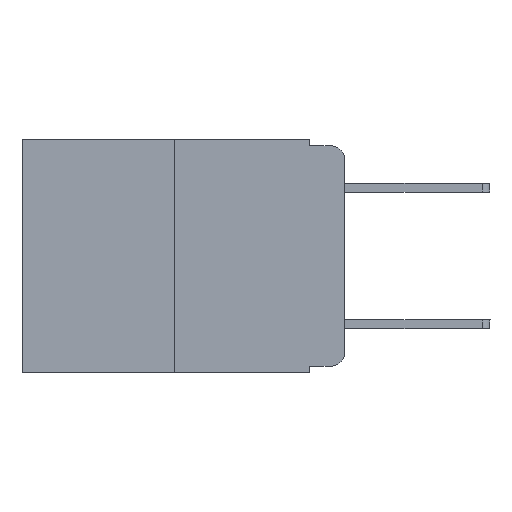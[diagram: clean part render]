
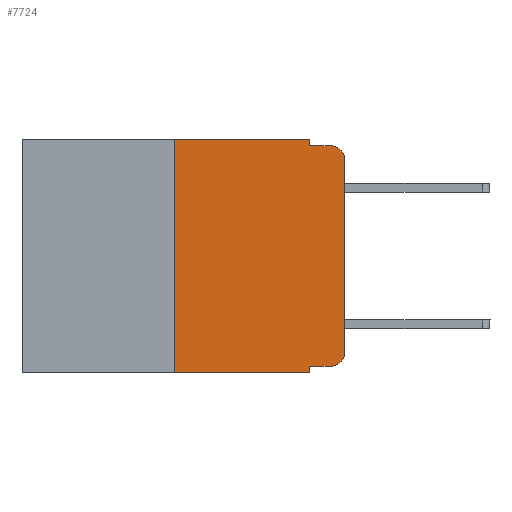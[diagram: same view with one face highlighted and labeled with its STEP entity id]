
A CAD part, left-side view. The second image highlights one B-rep face of the part: STEP entity #7724.
In plain terms, the highlighted planar face has unit normal (-1, 0, 0).
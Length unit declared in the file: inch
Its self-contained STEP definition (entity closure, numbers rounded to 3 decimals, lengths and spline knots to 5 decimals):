
#228 = CARTESIAN_POINT ( 'NONE',  ( 0., 0.02, -0.313 ) ) ;
#391 = LINE ( 'NONE', #3208, #10786 ) ;
#395 = LINE ( 'NONE', #9483, #9453 ) ;
#474 = EDGE_CURVE ( 'NONE', #6445, #5872, #391, .T. ) ;
#536 = VERTEX_POINT ( 'NONE', #8175 ) ;
#725 = DIRECTION ( 'NONE',  ( -1., 0., 0. ) ) ;
#826 = VERTEX_POINT ( 'NONE', #10182 ) ;
#1016 = ORIENTED_EDGE ( 'NONE', *, *, #15854, .T. ) ;
#1035 = VERTEX_POINT ( 'NONE', #9057 ) ;
#1087 = CARTESIAN_POINT ( 'NONE',  ( 0., 0.02, -0.01 ) ) ;
#1157 = CARTESIAN_POINT ( 'NONE',  ( 0., 0.473, -0.343 ) ) ;
#1328 = EDGE_CURVE ( 'NONE', #5872, #15276, #11912, .T. ) ;
#1641 = VERTEX_POINT ( 'NONE', #15728 ) ;
#1846 = ORIENTED_EDGE ( 'NONE', *, *, #10361, .T. ) ;
#1876 = LINE ( 'NONE', #10554, #15688 ) ;
#2297 = CARTESIAN_POINT ( 'NONE',  ( 0., 0.051, -0.01 ) ) ;
#3073 = DIRECTION ( 'NONE',  ( 1., 0., 0. ) ) ;
#3208 = CARTESIAN_POINT ( 'NONE',  ( 0., 0.25, 0. ) ) ;
#3392 = EDGE_CURVE ( 'NONE', #15276, #13575, #14019, .T. ) ;
#3909 = VECTOR ( 'NONE', #8403, 39.37008 ) ;
#4328 = DIRECTION ( 'NONE',  ( 0., 0., -1. ) ) ;
#4457 = DIRECTION ( 'NONE',  ( 0., 0., 1. ) ) ;
#4506 = DIRECTION ( 'NONE',  ( 0., -1., 0. ) ) ;
#4897 = DIRECTION ( 'NONE',  ( 0., 0., -1. ) ) ;
#4908 = EDGE_CURVE ( 'NONE', #8426, #826, #1876, .T. ) ;
#4985 = EDGE_CURVE ( 'NONE', #6445, #826, #8049, .T. ) ;
#5052 = ORIENTED_EDGE ( 'NONE', *, *, #10238, .T. ) ;
#5402 = VECTOR ( 'NONE', #4506, 39.37008 ) ;
#5697 = DIRECTION ( 'NONE',  ( 0., 0., -1. ) ) ;
#5754 = CARTESIAN_POINT ( 'NONE',  ( 0., 0.02, -0.03 ) ) ;
#5872 = VERTEX_POINT ( 'NONE', #8895 ) ;
#6039 = DIRECTION ( 'NONE',  ( 0., -1., 0. ) ) ;
#6445 = VERTEX_POINT ( 'NONE', #8767 ) ;
#6528 = VECTOR ( 'NONE', #6039, 39.37008 ) ;
#6930 = AXIS2_PLACEMENT_3D ( 'NONE', #11641, #3073, #4328 ) ;
#7294 = CIRCLE ( 'NONE', #13881, 0.02 ) ;
#7634 = LINE ( 'NONE', #13775, #11846 ) ;
#7724 = ADVANCED_FACE ( 'NONE', ( #15801 ), #10383, .F. ) ;
#7954 = EDGE_CURVE ( 'NONE', #13575, #13492, #14842, .T. ) ;
#8049 = LINE ( 'NONE', #1157, #6528 ) ;
#8175 = CARTESIAN_POINT ( 'NONE',  ( 0., 0.02, -0.333 ) ) ;
#8403 = DIRECTION ( 'NONE',  ( 0., -1., 0. ) ) ;
#8426 = VERTEX_POINT ( 'NONE', #15736 ) ;
#8454 = CARTESIAN_POINT ( 'NONE',  ( 0., 0.051, -0.01 ) ) ;
#8767 = CARTESIAN_POINT ( 'NONE',  ( 0., 0.25, -0.343 ) ) ;
#8841 = DIRECTION ( 'NONE',  ( -1., 0., 0. ) ) ;
#8895 = CARTESIAN_POINT ( 'NONE',  ( 0., 0.25, 0. ) ) ;
#9057 = CARTESIAN_POINT ( 'NONE',  ( 0., 0., -0.313 ) ) ;
#9325 = DIRECTION ( 'NONE',  ( 0., 0., 1. ) ) ;
#9336 = ORIENTED_EDGE ( 'NONE', *, *, #4908, .F. ) ;
#9453 = VECTOR ( 'NONE', #9325, 39.37008 ) ;
#9483 = CARTESIAN_POINT ( 'NONE',  ( 0., 0., 0. ) ) ;
#9988 = CARTESIAN_POINT ( 'NONE',  ( 0., 0.051, 0. ) ) ;
#10182 = CARTESIAN_POINT ( 'NONE',  ( 0., 0.051, -0.343 ) ) ;
#10238 = EDGE_CURVE ( 'NONE', #536, #1035, #12064, .T. ) ;
#10361 = EDGE_CURVE ( 'NONE', #1641, #13492, #7294, .T. ) ;
#10383 = PLANE ( 'NONE',  #6930 ) ;
#10502 = CARTESIAN_POINT ( 'NONE',  ( 0., 0.473, 0. ) ) ;
#10554 = CARTESIAN_POINT ( 'NONE',  ( 0., 0.051, 0. ) ) ;
#10778 = VECTOR ( 'NONE', #13101, 39.37008 ) ;
#10786 = VECTOR ( 'NONE', #4457, 39.37008 ) ;
#10828 = EDGE_CURVE ( 'NONE', #8426, #536, #7634, .T. ) ;
#10937 = ORIENTED_EDGE ( 'NONE', *, *, #7954, .F. ) ;
#11266 = DIRECTION ( 'NONE',  ( 0., 0., -1. ) ) ;
#11641 = CARTESIAN_POINT ( 'NONE',  ( 0., 0.473, 0. ) ) ;
#11743 = AXIS2_PLACEMENT_3D ( 'NONE', #228, #8841, #11266 ) ;
#11846 = VECTOR ( 'NONE', #12720, 39.37008 ) ;
#11912 = LINE ( 'NONE', #10502, #5402 ) ;
#12064 = CIRCLE ( 'NONE', #11743, 0.02 ) ;
#12537 = ORIENTED_EDGE ( 'NONE', *, *, #474, .F. ) ;
#12720 = DIRECTION ( 'NONE',  ( 0., -1., 0. ) ) ;
#12936 = ORIENTED_EDGE ( 'NONE', *, *, #1328, .F. ) ;
#13030 = ORIENTED_EDGE ( 'NONE', *, *, #3392, .F. ) ;
#13101 = DIRECTION ( 'NONE',  ( 0., 0., -1. ) ) ;
#13256 = CARTESIAN_POINT ( 'NONE',  ( 0., 0.051, 0. ) ) ;
#13492 = VERTEX_POINT ( 'NONE', #1087 ) ;
#13575 = VERTEX_POINT ( 'NONE', #2297 ) ;
#13775 = CARTESIAN_POINT ( 'NONE',  ( 0., 0.051, -0.333 ) ) ;
#13858 = EDGE_LOOP ( 'NONE', ( #1016, #1846, #10937, #13030, #12936, #12537, #14459, #9336, #13877, #5052 ) ) ;
#13877 = ORIENTED_EDGE ( 'NONE', *, *, #10828, .T. ) ;
#13881 = AXIS2_PLACEMENT_3D ( 'NONE', #5754, #725, #5697 ) ;
#14019 = LINE ( 'NONE', #13256, #10778 ) ;
#14459 = ORIENTED_EDGE ( 'NONE', *, *, #4985, .T. ) ;
#14842 = LINE ( 'NONE', #8454, #3909 ) ;
#15276 = VERTEX_POINT ( 'NONE', #9988 ) ;
#15688 = VECTOR ( 'NONE', #4897, 39.37008 ) ;
#15728 = CARTESIAN_POINT ( 'NONE',  ( 0., 0., -0.03 ) ) ;
#15736 = CARTESIAN_POINT ( 'NONE',  ( 0., 0.051, -0.333 ) ) ;
#15801 = FACE_OUTER_BOUND ( 'NONE', #13858, .T. ) ;
#15854 = EDGE_CURVE ( 'NONE', #1035, #1641, #395, .T. ) ;
